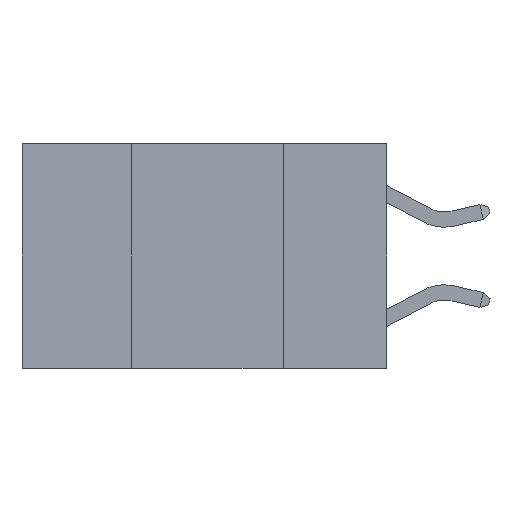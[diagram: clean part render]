
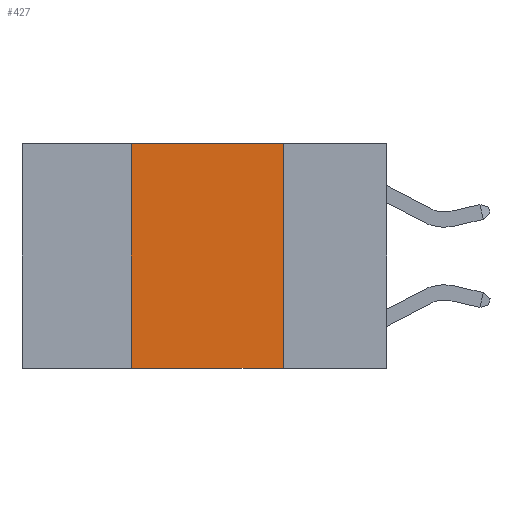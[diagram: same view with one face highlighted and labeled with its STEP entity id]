
A CAD part, left-side view. The second image highlights one B-rep face of the part: STEP entity #427.
In plain terms, the highlighted planar face has unit normal (-1, 0, 0).
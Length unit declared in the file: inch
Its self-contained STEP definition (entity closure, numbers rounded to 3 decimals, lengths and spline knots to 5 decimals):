
#427 = ADVANCED_FACE ( 'NONE', ( #12591 ), #18025, .F. ) ;
#574 = DIRECTION ( 'NONE',  ( 0., 0., 1. ) ) ;
#1277 = CARTESIAN_POINT ( 'NONE',  ( 0., 0.42, 0. ) ) ;
#2546 = EDGE_CURVE ( 'NONE', #9896, #26907, #17239, .T. ) ;
#2714 = DIRECTION ( 'NONE',  ( 0., 0., -1. ) ) ;
#4251 = CARTESIAN_POINT ( 'NONE',  ( 0., 0.42, -0.37 ) ) ;
#5968 = CARTESIAN_POINT ( 'NONE',  ( 0., 0.6, -0.37 ) ) ;
#6148 = CARTESIAN_POINT ( 'NONE',  ( 0., 0.6, 0. ) ) ;
#6794 = ORIENTED_EDGE ( 'NONE', *, *, #24491, .F. ) ;
#7504 = ORIENTED_EDGE ( 'NONE', *, *, #23547, .F. ) ;
#7831 = ORIENTED_EDGE ( 'NONE', *, *, #17858, .T. ) ;
#9382 = CARTESIAN_POINT ( 'NONE',  ( 0., 0.6, 0. ) ) ;
#9478 = DIRECTION ( 'NONE',  ( 0., 0., -1. ) ) ;
#9896 = VERTEX_POINT ( 'NONE', #4251 ) ;
#10096 = VECTOR ( 'NONE', #17048, 39.37008 ) ;
#10831 = VECTOR ( 'NONE', #9478, 39.37008 ) ;
#10889 = AXIS2_PLACEMENT_3D ( 'NONE', #9382, #15956, #2714 ) ;
#11827 = VECTOR ( 'NONE', #23297, 39.37008 ) ;
#12591 = FACE_OUTER_BOUND ( 'NONE', #26614, .T. ) ;
#13951 = CARTESIAN_POINT ( 'NONE',  ( 0., 0.17, 0. ) ) ;
#15908 = LINE ( 'NONE', #22281, #10831 ) ;
#15956 = DIRECTION ( 'NONE',  ( 1., 0., 0. ) ) ;
#17048 = DIRECTION ( 'NONE',  ( 0., -1., 0. ) ) ;
#17239 = LINE ( 'NONE', #22436, #27902 ) ;
#17858 = EDGE_CURVE ( 'NONE', #9896, #18729, #28184, .T. ) ;
#18025 = PLANE ( 'NONE',  #10889 ) ;
#18729 = VERTEX_POINT ( 'NONE', #19101 ) ;
#19101 = CARTESIAN_POINT ( 'NONE',  ( 0., 0.17, -0.37 ) ) ;
#21508 = LINE ( 'NONE', #6148, #10096 ) ;
#22281 = CARTESIAN_POINT ( 'NONE',  ( 0., 0.17, 0. ) ) ;
#22436 = CARTESIAN_POINT ( 'NONE',  ( 0., 0.42, 0. ) ) ;
#23297 = DIRECTION ( 'NONE',  ( 0., -1., 0. ) ) ;
#23547 = EDGE_CURVE ( 'NONE', #24329, #18729, #15908, .T. ) ;
#24000 = ORIENTED_EDGE ( 'NONE', *, *, #2546, .F. ) ;
#24329 = VERTEX_POINT ( 'NONE', #13951 ) ;
#24491 = EDGE_CURVE ( 'NONE', #26907, #24329, #21508, .T. ) ;
#26614 = EDGE_LOOP ( 'NONE', ( #7504, #6794, #24000, #7831 ) ) ;
#26907 = VERTEX_POINT ( 'NONE', #1277 ) ;
#27902 = VECTOR ( 'NONE', #574, 39.37008 ) ;
#28184 = LINE ( 'NONE', #5968, #11827 ) ;
